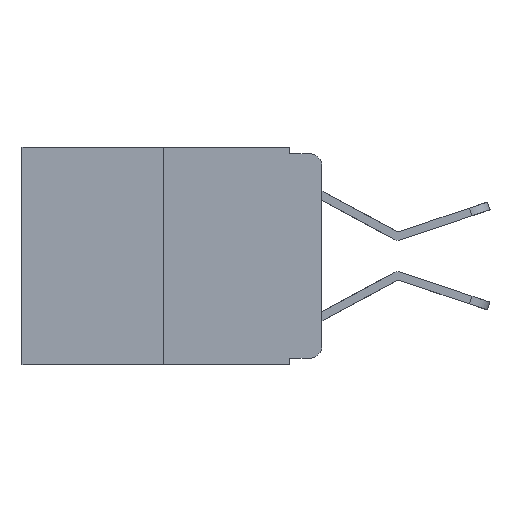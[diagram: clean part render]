
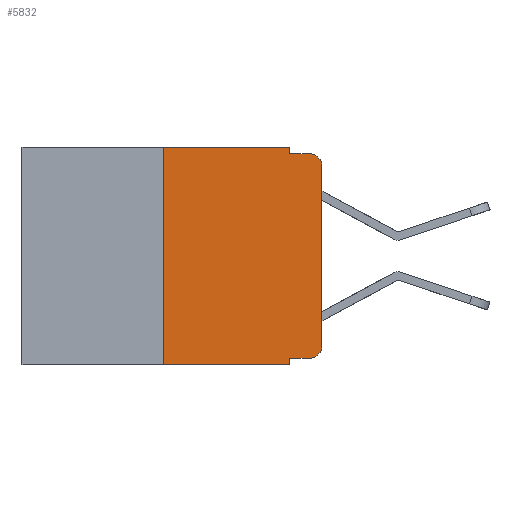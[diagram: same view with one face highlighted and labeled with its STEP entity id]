
A CAD part, left-side view. The second image highlights one B-rep face of the part: STEP entity #5832.
In plain terms, the highlighted planar face has unit normal (-1, 0, 0).
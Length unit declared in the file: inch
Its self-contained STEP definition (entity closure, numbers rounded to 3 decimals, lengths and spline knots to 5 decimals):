
#366 = CARTESIAN_POINT ( 'NONE',  ( 0., 0.25, 0. ) ) ;
#525 = CARTESIAN_POINT ( 'NONE',  ( 0., 0.02, -0.01 ) ) ;
#568 = VERTEX_POINT ( 'NONE', #2662 ) ;
#970 = ORIENTED_EDGE ( 'NONE', *, *, #15569, .T. ) ;
#1037 = EDGE_CURVE ( 'NONE', #6294, #11266, #11182, .T. ) ;
#1823 = DIRECTION ( 'NONE',  ( 0., -1., 0. ) ) ;
#1850 = VECTOR ( 'NONE', #19074, 39.37008 ) ;
#1932 = DIRECTION ( 'NONE',  ( 0., 0., -1. ) ) ;
#1996 = VECTOR ( 'NONE', #20837, 39.37008 ) ;
#2653 = FACE_OUTER_BOUND ( 'NONE', #18693, .T. ) ;
#2662 = CARTESIAN_POINT ( 'NONE',  ( 0., 0.051, -0.01 ) ) ;
#3428 = AXIS2_PLACEMENT_3D ( 'NONE', #4272, #12742, #19629 ) ;
#4114 = CARTESIAN_POINT ( 'NONE',  ( 0., 0.051, -0.333 ) ) ;
#4272 = CARTESIAN_POINT ( 'NONE',  ( 0., 0.473, 0. ) ) ;
#4390 = CARTESIAN_POINT ( 'NONE',  ( 0., 0., 0. ) ) ;
#4488 = CARTESIAN_POINT ( 'NONE',  ( 0., 0.051, -0.01 ) ) ;
#4811 = LINE ( 'NONE', #12629, #17782 ) ;
#4890 = CARTESIAN_POINT ( 'NONE',  ( 0., 0.02, -0.03 ) ) ;
#5091 = CARTESIAN_POINT ( 'NONE',  ( 0., 0.02, -0.333 ) ) ;
#5598 = VECTOR ( 'NONE', #22472, 39.37008 ) ;
#5832 = ADVANCED_FACE ( 'NONE', ( #2653 ), #17853, .F. ) ;
#6294 = VERTEX_POINT ( 'NONE', #10043 ) ;
#6299 = DIRECTION ( 'NONE',  ( 0., -1., 0. ) ) ;
#6349 = VERTEX_POINT ( 'NONE', #5091 ) ;
#6649 = DIRECTION ( 'NONE',  ( 0., 0., -1. ) ) ;
#7284 = VERTEX_POINT ( 'NONE', #366 ) ;
#7542 = CIRCLE ( 'NONE', #18325, 0.02 ) ;
#7773 = VERTEX_POINT ( 'NONE', #4114 ) ;
#7872 = DIRECTION ( 'NONE',  ( 0., 0., 1. ) ) ;
#8686 = AXIS2_PLACEMENT_3D ( 'NONE', #9987, #21848, #11654 ) ;
#8894 = EDGE_CURVE ( 'NONE', #7773, #11266, #14546, .T. ) ;
#8898 = CARTESIAN_POINT ( 'NONE',  ( 0., 0.473, 0. ) ) ;
#9861 = EDGE_CURVE ( 'NONE', #18734, #16756, #15734, .T. ) ;
#9987 = CARTESIAN_POINT ( 'NONE',  ( 0., 0.02, -0.313 ) ) ;
#10043 = CARTESIAN_POINT ( 'NONE',  ( 0., 0.25, -0.343 ) ) ;
#10188 = VECTOR ( 'NONE', #1932, 39.37008 ) ;
#10212 = VECTOR ( 'NONE', #6299, 39.37008 ) ;
#10689 = CARTESIAN_POINT ( 'NONE',  ( 0., 0.051, -0.333 ) ) ;
#10763 = ORIENTED_EDGE ( 'NONE', *, *, #14742, .T. ) ;
#11182 = LINE ( 'NONE', #21604, #1850 ) ;
#11266 = VERTEX_POINT ( 'NONE', #12142 ) ;
#11654 = DIRECTION ( 'NONE',  ( 0., 0., -1. ) ) ;
#12112 = VECTOR ( 'NONE', #1823, 39.37008 ) ;
#12142 = CARTESIAN_POINT ( 'NONE',  ( 0., 0.051, -0.343 ) ) ;
#12565 = VERTEX_POINT ( 'NONE', #525 ) ;
#12629 = CARTESIAN_POINT ( 'NONE',  ( 0., 0.051, 0. ) ) ;
#12742 = DIRECTION ( 'NONE',  ( 1., 0., 0. ) ) ;
#13316 = EDGE_CURVE ( 'NONE', #13781, #568, #4811, .T. ) ;
#13781 = VERTEX_POINT ( 'NONE', #18960 ) ;
#13929 = CARTESIAN_POINT ( 'NONE',  ( 0., 0., -0.313 ) ) ;
#13974 = LINE ( 'NONE', #8898, #5598 ) ;
#14133 = DIRECTION ( 'NONE',  ( 0., 0., -1. ) ) ;
#14340 = EDGE_CURVE ( 'NONE', #7284, #13781, #13974, .T. ) ;
#14546 = LINE ( 'NONE', #22583, #10188 ) ;
#14742 = EDGE_CURVE ( 'NONE', #6349, #18734, #19092, .T. ) ;
#15086 = LINE ( 'NONE', #4488, #10212 ) ;
#15569 = EDGE_CURVE ( 'NONE', #7773, #6349, #20659, .T. ) ;
#15734 = LINE ( 'NONE', #4390, #19316 ) ;
#15835 = ORIENTED_EDGE ( 'NONE', *, *, #16257, .F. ) ;
#15961 = ORIENTED_EDGE ( 'NONE', *, *, #14340, .F. ) ;
#16148 = ORIENTED_EDGE ( 'NONE', *, *, #13316, .F. ) ;
#16187 = ORIENTED_EDGE ( 'NONE', *, *, #18329, .F. ) ;
#16257 = EDGE_CURVE ( 'NONE', #6294, #7284, #20358, .T. ) ;
#16667 = DIRECTION ( 'NONE',  ( -1., 0., 0. ) ) ;
#16686 = ORIENTED_EDGE ( 'NONE', *, *, #9861, .T. ) ;
#16756 = VERTEX_POINT ( 'NONE', #18832 ) ;
#17309 = CARTESIAN_POINT ( 'NONE',  ( 0., 0.25, 0. ) ) ;
#17782 = VECTOR ( 'NONE', #14133, 39.37008 ) ;
#17853 = PLANE ( 'NONE',  #3428 ) ;
#18325 = AXIS2_PLACEMENT_3D ( 'NONE', #4890, #16667, #6649 ) ;
#18329 = EDGE_CURVE ( 'NONE', #568, #12565, #15086, .T. ) ;
#18472 = EDGE_CURVE ( 'NONE', #16756, #12565, #7542, .T. ) ;
#18693 = EDGE_LOOP ( 'NONE', ( #16686, #20547, #16187, #16148, #15961, #15835, #22133, #21051, #970, #10763 ) ) ;
#18734 = VERTEX_POINT ( 'NONE', #13929 ) ;
#18832 = CARTESIAN_POINT ( 'NONE',  ( 0., 0., -0.03 ) ) ;
#18960 = CARTESIAN_POINT ( 'NONE',  ( 0., 0.051, 0. ) ) ;
#19074 = DIRECTION ( 'NONE',  ( 0., -1., 0. ) ) ;
#19092 = CIRCLE ( 'NONE', #8686, 0.02 ) ;
#19316 = VECTOR ( 'NONE', #7872, 39.37008 ) ;
#19629 = DIRECTION ( 'NONE',  ( 0., 0., -1. ) ) ;
#20358 = LINE ( 'NONE', #17309, #1996 ) ;
#20547 = ORIENTED_EDGE ( 'NONE', *, *, #18472, .T. ) ;
#20659 = LINE ( 'NONE', #10689, #12112 ) ;
#20837 = DIRECTION ( 'NONE',  ( 0., 0., 1. ) ) ;
#21051 = ORIENTED_EDGE ( 'NONE', *, *, #8894, .F. ) ;
#21604 = CARTESIAN_POINT ( 'NONE',  ( 0., 0.473, -0.343 ) ) ;
#21848 = DIRECTION ( 'NONE',  ( -1., 0., 0. ) ) ;
#22133 = ORIENTED_EDGE ( 'NONE', *, *, #1037, .T. ) ;
#22472 = DIRECTION ( 'NONE',  ( 0., -1., 0. ) ) ;
#22583 = CARTESIAN_POINT ( 'NONE',  ( 0., 0.051, 0. ) ) ;
